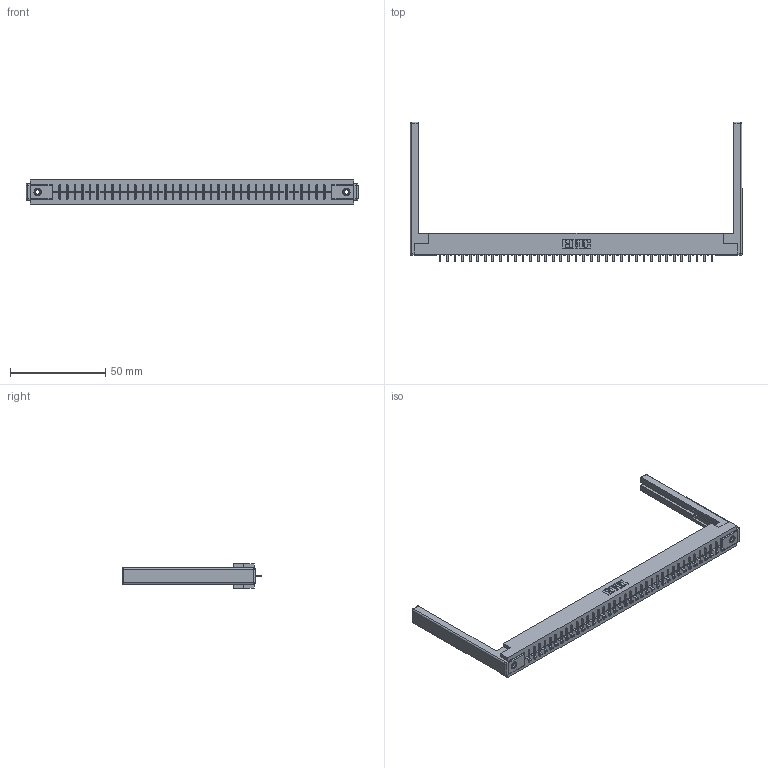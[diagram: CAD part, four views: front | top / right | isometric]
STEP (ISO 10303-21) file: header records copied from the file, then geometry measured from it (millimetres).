
FILE_DESCRIPTION (( 'STEP AP203' ), '1' );
FILE_NAME ('356-037-421-168.STEP', '2020-09-23T23:27:49', ( '' ), ( '' ), 'SwSTEP 2.0', 'SolidWorks 2020', '' );
FILE_SCHEMA (( 'CONFIG_CONTROL_DESIGN' ));
Length unit declared in the file: inch
Products named in the file (5): 306 Part_.156 Dia; 306-290-001_121; 356-037-421-168; 307-220-068; 345-250-001_345-250-001-102
Assembly tree (42 placements, depth 2):
  356-037-421-168
    306 Part_.156 Dia
    306-290-001_121  x37
    345-250-001_345-250-001-102  x2
    307-220-068  x2
Bounding box: 174.04 x 73.18 x 12.7 mm (x, y, z)
Volume: 23514.5 mm3; surface area: 23397.4 mm2
Topology: 42 solids, 42 shells, 2860 faces, 7995 edges, 5110 vertices
Faces by surface type: plane 1895, cylinder 793, sphere 156, cone 12, torus 4
Entity records: 37867 total; most frequent: CARTESIAN_POINT 6323, ORIENTED_EDGE 6260, DIRECTION 6248, EDGE_CURVE 3130, VECTOR 2442, LINE 2442, VERTEX_POINT 1978, AXIS2_PLACEMENT_3D 1903
